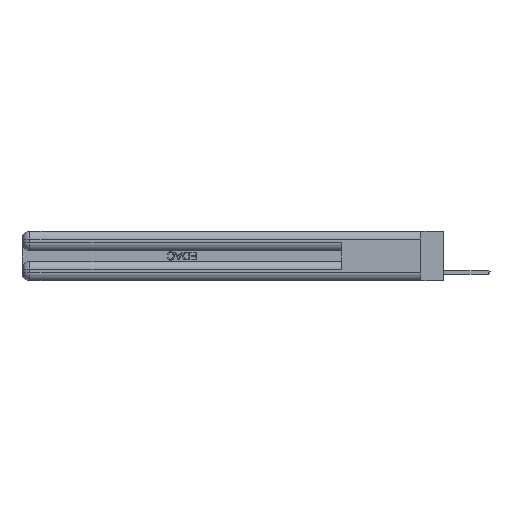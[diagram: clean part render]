
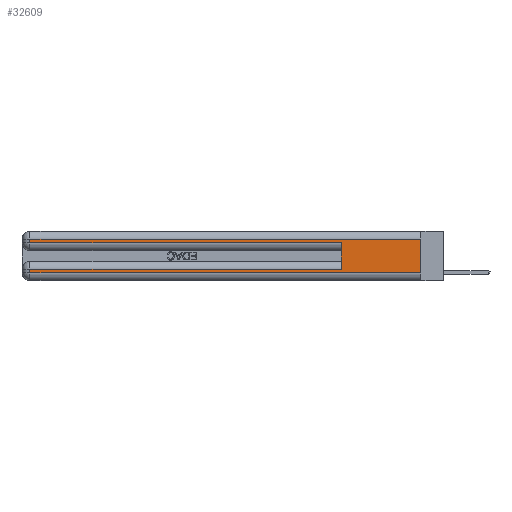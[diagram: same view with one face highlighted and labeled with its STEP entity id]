
A CAD part, left-side view. The second image highlights one B-rep face of the part: STEP entity #32609.
In plain terms, the highlighted planar face has unit normal (-1, 0, 0).
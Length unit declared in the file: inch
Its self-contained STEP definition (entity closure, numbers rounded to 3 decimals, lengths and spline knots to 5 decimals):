
#846 = VERTEX_POINT ( 'NONE', #15431 ) ;
#1889 = DIRECTION ( 'NONE',  ( 0., -1., 0. ) ) ;
#1954 = DIRECTION ( 'NONE',  ( 0., -1., 0. ) ) ;
#2657 = VECTOR ( 'NONE', #20625, 39.37008 ) ;
#2904 = CARTESIAN_POINT ( 'NONE',  ( 0., 2.94, 0.085 ) ) ;
#4019 = DIRECTION ( 'NONE',  ( 0., 1., 0. ) ) ;
#4489 = CARTESIAN_POINT ( 'NONE',  ( 0., 2.94, 0.31 ) ) ;
#4506 = DIRECTION ( 'NONE',  ( 1., 0., 0. ) ) ;
#4736 = CARTESIAN_POINT ( 'NONE',  ( 0., 0., 0.37 ) ) ;
#5742 = VERTEX_POINT ( 'NONE', #14002 ) ;
#5920 = EDGE_CURVE ( 'NONE', #28065, #846, #12768, .T. ) ;
#6125 = EDGE_CURVE ( 'NONE', #31733, #6766, #24518, .T. ) ;
#6733 = ORIENTED_EDGE ( 'NONE', *, *, #6125, .T. ) ;
#6766 = VERTEX_POINT ( 'NONE', #15075 ) ;
#7377 = CARTESIAN_POINT ( 'NONE',  ( 0., 0., 0.06 ) ) ;
#8162 = ORIENTED_EDGE ( 'NONE', *, *, #11555, .F. ) ;
#9087 = CARTESIAN_POINT ( 'NONE',  ( 0., 0., 0.31 ) ) ;
#9563 = AXIS2_PLACEMENT_3D ( 'NONE', #4736, #4506, #33879 ) ;
#9835 = LINE ( 'NONE', #25034, #11515 ) ;
#11209 = ORIENTED_EDGE ( 'NONE', *, *, #16381, .T. ) ;
#11515 = VECTOR ( 'NONE', #30423, 39.37008 ) ;
#11555 = EDGE_CURVE ( 'NONE', #5742, #30114, #9835, .T. ) ;
#12074 = EDGE_CURVE ( 'NONE', #5742, #31733, #27083, .T. ) ;
#12768 = LINE ( 'NONE', #15305, #23694 ) ;
#13541 = CARTESIAN_POINT ( 'NONE',  ( 0., 0.6, 0.285 ) ) ;
#13571 = DIRECTION ( 'NONE',  ( 0., 1., 0. ) ) ;
#13661 = EDGE_CURVE ( 'NONE', #22577, #28065, #21075, .T. ) ;
#14002 = CARTESIAN_POINT ( 'NONE',  ( 0., 0.6, 0.085 ) ) ;
#14266 = EDGE_LOOP ( 'NONE', ( #28494, #20682, #18473, #11209, #8162, #15573, #6733, #26886 ) ) ;
#15075 = CARTESIAN_POINT ( 'NONE',  ( 0., 2.94, 0.06 ) ) ;
#15305 = CARTESIAN_POINT ( 'NONE',  ( 0., 2.94, 0.37 ) ) ;
#15431 = CARTESIAN_POINT ( 'NONE',  ( 0., 2.94, 0.285 ) ) ;
#15573 = ORIENTED_EDGE ( 'NONE', *, *, #12074, .T. ) ;
#16381 = EDGE_CURVE ( 'NONE', #846, #30114, #24169, .T. ) ;
#16850 = EDGE_CURVE ( 'NONE', #6766, #21976, #29562, .T. ) ;
#17023 = VECTOR ( 'NONE', #1889, 39.37008 ) ;
#18380 = LINE ( 'NONE', #26453, #19177 ) ;
#18473 = ORIENTED_EDGE ( 'NONE', *, *, #5920, .T. ) ;
#19177 = VECTOR ( 'NONE', #29843, 39.37008 ) ;
#20625 = DIRECTION ( 'NONE',  ( 0., 0., -1. ) ) ;
#20682 = ORIENTED_EDGE ( 'NONE', *, *, #13661, .T. ) ;
#21075 = LINE ( 'NONE', #9087, #34098 ) ;
#21797 = CARTESIAN_POINT ( 'NONE',  ( 0., 0., 0.085 ) ) ;
#21976 = VERTEX_POINT ( 'NONE', #24433 ) ;
#22577 = VERTEX_POINT ( 'NONE', #29976 ) ;
#23694 = VECTOR ( 'NONE', #26132, 39.37008 ) ;
#24169 = LINE ( 'NONE', #28686, #17023 ) ;
#24433 = CARTESIAN_POINT ( 'NONE',  ( 0., 0., 0.06 ) ) ;
#24518 = LINE ( 'NONE', #34018, #2657 ) ;
#25034 = CARTESIAN_POINT ( 'NONE',  ( 0., 0.6, 0.145 ) ) ;
#25417 = VECTOR ( 'NONE', #13571, 39.37008 ) ;
#26132 = DIRECTION ( 'NONE',  ( 0., 0., -1. ) ) ;
#26343 = EDGE_CURVE ( 'NONE', #22577, #21976, #18380, .T. ) ;
#26453 = CARTESIAN_POINT ( 'NONE',  ( 0., 0., 0.37 ) ) ;
#26886 = ORIENTED_EDGE ( 'NONE', *, *, #16850, .T. ) ;
#27083 = LINE ( 'NONE', #21797, #25417 ) ;
#28065 = VERTEX_POINT ( 'NONE', #4489 ) ;
#28494 = ORIENTED_EDGE ( 'NONE', *, *, #26343, .F. ) ;
#28686 = CARTESIAN_POINT ( 'NONE',  ( 0., 0., 0.285 ) ) ;
#29562 = LINE ( 'NONE', #7377, #33771 ) ;
#29843 = DIRECTION ( 'NONE',  ( 0., 0., -1. ) ) ;
#29976 = CARTESIAN_POINT ( 'NONE',  ( 0., 0., 0.31 ) ) ;
#30114 = VERTEX_POINT ( 'NONE', #13541 ) ;
#30423 = DIRECTION ( 'NONE',  ( 0., 0., 1. ) ) ;
#30787 = FACE_OUTER_BOUND ( 'NONE', #14266, .T. ) ;
#31653 = PLANE ( 'NONE',  #9563 ) ;
#31733 = VERTEX_POINT ( 'NONE', #2904 ) ;
#32609 = ADVANCED_FACE ( 'NONE', ( #30787 ), #31653, .F. ) ;
#33771 = VECTOR ( 'NONE', #1954, 39.37008 ) ;
#33879 = DIRECTION ( 'NONE',  ( 0., 0., -1. ) ) ;
#34018 = CARTESIAN_POINT ( 'NONE',  ( 0., 2.94, 0.37 ) ) ;
#34098 = VECTOR ( 'NONE', #4019, 39.37008 ) ;
